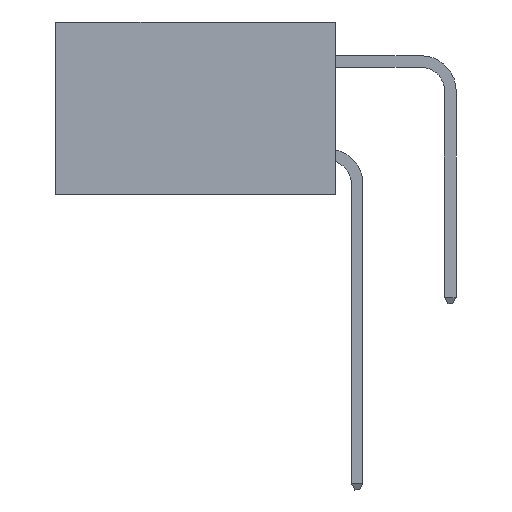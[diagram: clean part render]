
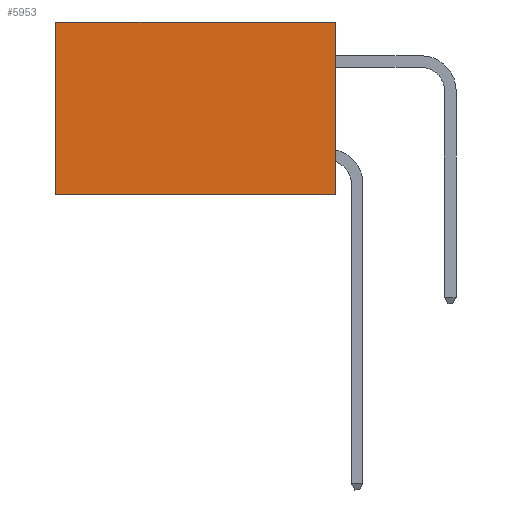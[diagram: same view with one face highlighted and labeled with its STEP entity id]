
A CAD part, left-side view. The second image highlights one B-rep face of the part: STEP entity #5953.
In plain terms, the highlighted planar face has unit normal (-1, 0, 0).
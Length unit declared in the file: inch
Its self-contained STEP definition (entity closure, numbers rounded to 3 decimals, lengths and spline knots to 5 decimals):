
#742 = ORIENTED_EDGE ( 'NONE', *, *, #8967, .F. ) ;
#858 = CARTESIAN_POINT ( 'NONE',  ( 0.2875, 0.6, 0. ) ) ;
#1383 = VERTEX_POINT ( 'NONE', #13404 ) ;
#2092 = VECTOR ( 'NONE', #22035, 39.37008 ) ;
#2975 = LINE ( 'NONE', #4376, #11274 ) ;
#3246 = CARTESIAN_POINT ( 'NONE',  ( 0.2875, 0., 0. ) ) ;
#4016 = AXIS2_PLACEMENT_3D ( 'NONE', #7487, #22637, #11304 ) ;
#4369 = LINE ( 'NONE', #19424, #13304 ) ;
#4376 = CARTESIAN_POINT ( 'NONE',  ( 0.2875, 0., 0. ) ) ;
#5309 = CARTESIAN_POINT ( 'NONE',  ( 0.2875, 0., 0. ) ) ;
#5953 = ADVANCED_FACE ( 'NONE', ( #24438 ), #18815, .F. ) ;
#6671 = EDGE_LOOP ( 'NONE', ( #18544, #742, #20762, #7815 ) ) ;
#6967 = DIRECTION ( 'NONE',  ( 0., 1., 0. ) ) ;
#7128 = VERTEX_POINT ( 'NONE', #23971 ) ;
#7487 = CARTESIAN_POINT ( 'NONE',  ( 0.2875, 0., 0. ) ) ;
#7815 = ORIENTED_EDGE ( 'NONE', *, *, #22181, .T. ) ;
#7953 = LINE ( 'NONE', #5309, #18301 ) ;
#8967 = EDGE_CURVE ( 'NONE', #1383, #7128, #4369, .T. ) ;
#9890 = VERTEX_POINT ( 'NONE', #858 ) ;
#11274 = VECTOR ( 'NONE', #6967, 39.37008 ) ;
#11304 = DIRECTION ( 'NONE',  ( 0., 0., -1. ) ) ;
#11643 = DIRECTION ( 'NONE',  ( 0., 1., 0. ) ) ;
#12790 = LINE ( 'NONE', #20746, #2092 ) ;
#13263 = VERTEX_POINT ( 'NONE', #3246 ) ;
#13304 = VECTOR ( 'NONE', #11643, 39.37008 ) ;
#13404 = CARTESIAN_POINT ( 'NONE',  ( 0.2875, 0., -0.37 ) ) ;
#13646 = EDGE_CURVE ( 'NONE', #9890, #7128, #12790, .T. ) ;
#16649 = DIRECTION ( 'NONE',  ( 0., 0., -1. ) ) ;
#18301 = VECTOR ( 'NONE', #16649, 39.37008 ) ;
#18544 = ORIENTED_EDGE ( 'NONE', *, *, #13646, .T. ) ;
#18815 = PLANE ( 'NONE',  #4016 ) ;
#19424 = CARTESIAN_POINT ( 'NONE',  ( 0.2875, 0., -0.37 ) ) ;
#20261 = EDGE_CURVE ( 'NONE', #13263, #1383, #7953, .T. ) ;
#20746 = CARTESIAN_POINT ( 'NONE',  ( 0.2875, 0.6, 0. ) ) ;
#20762 = ORIENTED_EDGE ( 'NONE', *, *, #20261, .F. ) ;
#22035 = DIRECTION ( 'NONE',  ( 0., 0., -1. ) ) ;
#22181 = EDGE_CURVE ( 'NONE', #13263, #9890, #2975, .T. ) ;
#22637 = DIRECTION ( 'NONE',  ( 1., 0., 0. ) ) ;
#23971 = CARTESIAN_POINT ( 'NONE',  ( 0.2875, 0.6, -0.37 ) ) ;
#24438 = FACE_OUTER_BOUND ( 'NONE', #6671, .T. ) ;
